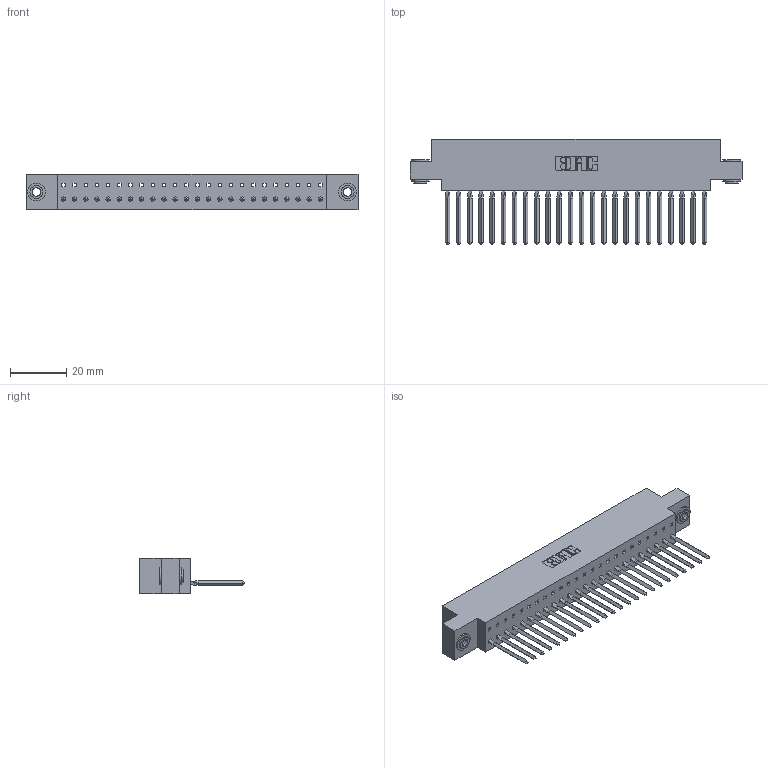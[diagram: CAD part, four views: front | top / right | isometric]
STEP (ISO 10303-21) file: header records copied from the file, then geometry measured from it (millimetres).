
FILE_DESCRIPTION (( 'STEP AP203' ), '1' );
FILE_NAME ('317-024-542-603.STEP', '2020-02-27T17:52:33', ( '' ), ( '' ), 'SwSTEP 2.0', 'SolidWorks 2016', '' );
FILE_SCHEMA (( 'CONFIG_CONTROL_DESIGN' ));
Length unit declared in the file: inch
Products named in the file (4): 317-290-003_542; 317 Part_.156 Dia - TH; 345-250-002_345-250-002-102; 317-024-542-603
Assembly tree (27 placements, depth 2):
  317-024-542-603
    317 Part_.156 Dia - TH
    317-290-003_542  x24
    345-250-002_345-250-002-102  x2
Bounding box: 117.81 x 37.34 x 12.7 mm (x, y, z)
Volume: 17738.5 mm3; surface area: 21457 mm2
Topology: 27 solids, 27 shells, 1940 faces, 5559 edges, 3590 vertices
Faces by surface type: plane 1604, cylinder 232, bspline 96, cone 8
Entity records: 36102 total; most frequent: CARTESIAN_POINT 6624, ORIENTED_EDGE 6304, DIRECTION 5326, EDGE_CURVE 3152, VECTOR 2958, LINE 2958, VERTEX_POINT 2094, AXIS2_PLACEMENT_3D 1184
